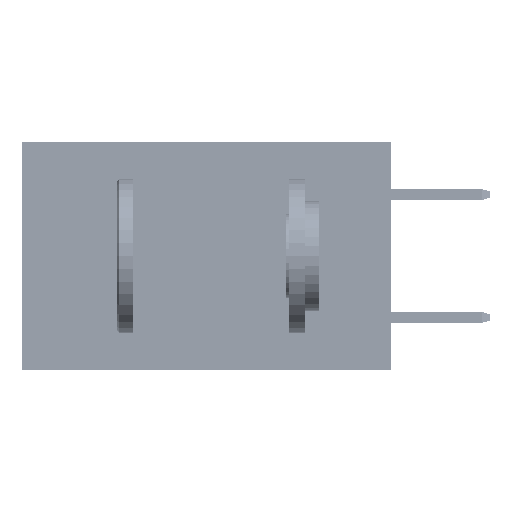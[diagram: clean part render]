
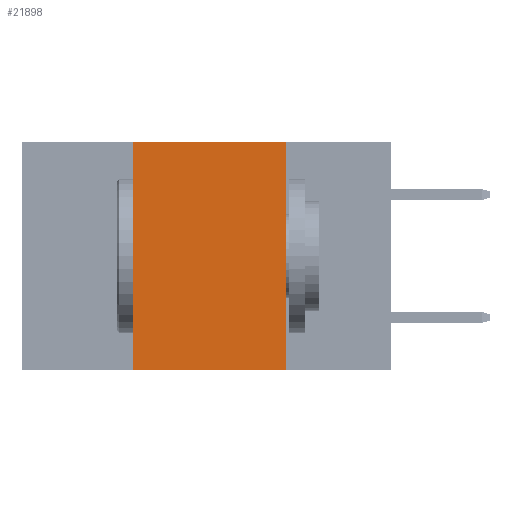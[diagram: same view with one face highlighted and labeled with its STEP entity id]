
A CAD part, left-side view. The second image highlights one B-rep face of the part: STEP entity #21898.
In plain terms, the highlighted planar face has unit normal (-1, 0, 0).
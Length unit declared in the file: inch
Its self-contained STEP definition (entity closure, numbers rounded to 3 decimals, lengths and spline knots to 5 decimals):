
#2878 = DIRECTION ( 'NONE',  ( 0., 0., -1. ) ) ;
#2995 = ORIENTED_EDGE ( 'NONE', *, *, #22258, .T. ) ;
#3879 = LINE ( 'NONE', #13901, #28897 ) ;
#4185 = CARTESIAN_POINT ( 'NONE',  ( 0., 0.6, -0.37 ) ) ;
#5835 = VECTOR ( 'NONE', #7924, 39.37008 ) ;
#6312 = DIRECTION ( 'NONE',  ( 1., 0., 0. ) ) ;
#7851 = LINE ( 'NONE', #9770, #11334 ) ;
#7924 = DIRECTION ( 'NONE',  ( 0., -1., 0. ) ) ;
#9770 = CARTESIAN_POINT ( 'NONE',  ( 0., 0.6, 0. ) ) ;
#11334 = VECTOR ( 'NONE', #42792, 39.37008 ) ;
#13310 = CARTESIAN_POINT ( 'NONE',  ( 0., 0.42, 0. ) ) ;
#13896 = EDGE_CURVE ( 'NONE', #27529, #25217, #18329, .T. ) ;
#13901 = CARTESIAN_POINT ( 'NONE',  ( 0., 0.17, 0. ) ) ;
#17375 = PLANE ( 'NONE',  #47168 ) ;
#18329 = LINE ( 'NONE', #13310, #40430 ) ;
#21466 = CARTESIAN_POINT ( 'NONE',  ( 0., 0.42, -0.37 ) ) ;
#21898 = ADVANCED_FACE ( 'NONE', ( #34406 ), #17375, .F. ) ;
#22258 = EDGE_CURVE ( 'NONE', #27529, #34020, #43623, .T. ) ;
#24353 = DIRECTION ( 'NONE',  ( 0., 0., -1. ) ) ;
#25217 = VERTEX_POINT ( 'NONE', #31157 ) ;
#27162 = EDGE_LOOP ( 'NONE', ( #47800, #37733, #27733, #2995 ) ) ;
#27529 = VERTEX_POINT ( 'NONE', #21466 ) ;
#27733 = ORIENTED_EDGE ( 'NONE', *, *, #13896, .F. ) ;
#28897 = VECTOR ( 'NONE', #2878, 39.37008 ) ;
#31157 = CARTESIAN_POINT ( 'NONE',  ( 0., 0.42, 0. ) ) ;
#31750 = VERTEX_POINT ( 'NONE', #48134 ) ;
#34020 = VERTEX_POINT ( 'NONE', #43389 ) ;
#34406 = FACE_OUTER_BOUND ( 'NONE', #27162, .T. ) ;
#37631 = EDGE_CURVE ( 'NONE', #31750, #34020, #3879, .T. ) ;
#37733 = ORIENTED_EDGE ( 'NONE', *, *, #40078, .F. ) ;
#39323 = CARTESIAN_POINT ( 'NONE',  ( 0., 0.6, 0. ) ) ;
#39339 = DIRECTION ( 'NONE',  ( 0., 0., 1. ) ) ;
#40078 = EDGE_CURVE ( 'NONE', #25217, #31750, #7851, .T. ) ;
#40430 = VECTOR ( 'NONE', #39339, 39.37008 ) ;
#42792 = DIRECTION ( 'NONE',  ( 0., -1., 0. ) ) ;
#43389 = CARTESIAN_POINT ( 'NONE',  ( 0., 0.17, -0.37 ) ) ;
#43623 = LINE ( 'NONE', #4185, #5835 ) ;
#47168 = AXIS2_PLACEMENT_3D ( 'NONE', #39323, #6312, #24353 ) ;
#47800 = ORIENTED_EDGE ( 'NONE', *, *, #37631, .F. ) ;
#48134 = CARTESIAN_POINT ( 'NONE',  ( 0., 0.17, 0. ) ) ;
